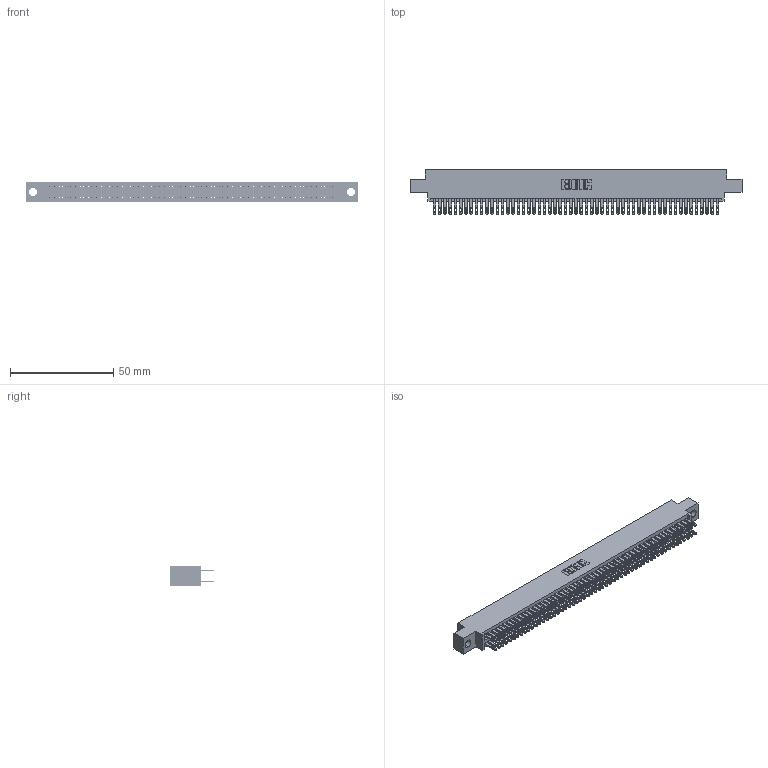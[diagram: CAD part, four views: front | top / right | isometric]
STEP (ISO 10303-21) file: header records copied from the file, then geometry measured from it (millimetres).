
FILE_DESCRIPTION (( 'STEP AP203' ), '1' );
FILE_NAME ('345-110-500-804.STEP', '2018-10-07T08:52:57', ( '' ), ( '' ), 'SwSTEP 2.0', 'SolidWorks 2016', '' );
FILE_SCHEMA (( 'CONFIG_CONTROL_DESIGN' ));
Length unit declared in the file: inch
Products named in the file (3): 345-110-500-804; 345 Part_0.170 Offset - 0.156 Dia-TH; 345-292-001_345-293-100
Assembly tree (111 placements, depth 2):
  345-110-500-804
    345 Part_0.170 Offset - 0.156 Dia-TH
    345-292-001_345-293-100  x110
Bounding box: 160.91 x 21.51 x 9.4 mm (x, y, z)
Volume: 15886.4 mm3; surface area: 24815.2 mm2
Topology: 111 solids, 111 shells, 5190 faces, 15863 edges, 10574 vertices
Faces by surface type: plane 3054, cylinder 2136
Entity records: 41469 total; most frequent: CARTESIAN_POINT 6940, ORIENTED_EDGE 6874, DIRECTION 6105, EDGE_CURVE 3437, LINE 3081, VECTOR 3081, VERTEX_POINT 2290, AXIS2_PLACEMENT_3D 1512
